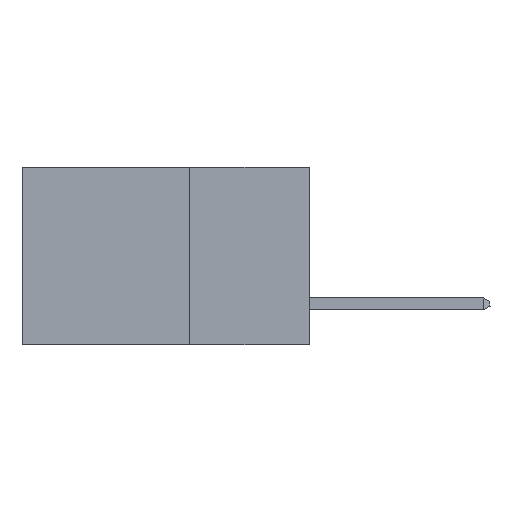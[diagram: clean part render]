
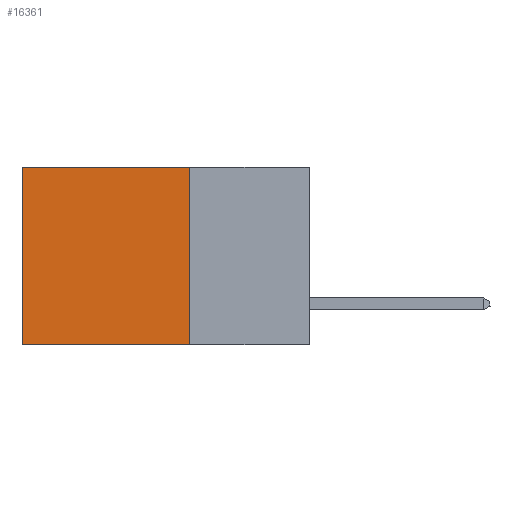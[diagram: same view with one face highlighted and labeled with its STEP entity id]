
A CAD part, left-side view. The second image highlights one B-rep face of the part: STEP entity #16361.
In plain terms, the highlighted planar face has unit normal (-1, 0, 0).
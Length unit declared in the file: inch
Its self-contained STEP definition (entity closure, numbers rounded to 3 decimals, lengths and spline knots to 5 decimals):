
#783 = VECTOR ( 'NONE', #18225, 39.37008 ) ;
#1828 = VERTEX_POINT ( 'NONE', #3755 ) ;
#2217 = EDGE_CURVE ( 'NONE', #1828, #13126, #6902, .T. ) ;
#2695 = DIRECTION ( 'NONE',  ( 0., 0., -1. ) ) ;
#3755 = CARTESIAN_POINT ( 'NONE',  ( 0.2875, 0.25, 0. ) ) ;
#3832 = ORIENTED_EDGE ( 'NONE', *, *, #2217, .F. ) ;
#5717 = EDGE_CURVE ( 'NONE', #6913, #8859, #11396, .T. ) ;
#6776 = AXIS2_PLACEMENT_3D ( 'NONE', #12167, #13519, #13450 ) ;
#6842 = DIRECTION ( 'NONE',  ( 0., 0., -1. ) ) ;
#6902 = LINE ( 'NONE', #15708, #10054 ) ;
#6913 = VERTEX_POINT ( 'NONE', #17330 ) ;
#7118 = EDGE_CURVE ( 'NONE', #1828, #6913, #10706, .T. ) ;
#8121 = CARTESIAN_POINT ( 'NONE',  ( 0.2875, 0.25, -0.37 ) ) ;
#8601 = ORIENTED_EDGE ( 'NONE', *, *, #5717, .T. ) ;
#8713 = LINE ( 'NONE', #9510, #14536 ) ;
#8859 = VERTEX_POINT ( 'NONE', #9231 ) ;
#9231 = CARTESIAN_POINT ( 'NONE',  ( 0.2875, 0.6, -0.37 ) ) ;
#9510 = CARTESIAN_POINT ( 'NONE',  ( 0.2875, 0.25, -0.37 ) ) ;
#10054 = VECTOR ( 'NONE', #2695, 39.37008 ) ;
#10706 = LINE ( 'NONE', #13238, #783 ) ;
#11093 = DIRECTION ( 'NONE',  ( 0., 1., 0. ) ) ;
#11351 = ORIENTED_EDGE ( 'NONE', *, *, #7118, .T. ) ;
#11396 = LINE ( 'NONE', #16739, #17244 ) ;
#12167 = CARTESIAN_POINT ( 'NONE',  ( 0.2875, 0.25, 0. ) ) ;
#13126 = VERTEX_POINT ( 'NONE', #8121 ) ;
#13238 = CARTESIAN_POINT ( 'NONE',  ( 0.2875, 0.25, 0. ) ) ;
#13450 = DIRECTION ( 'NONE',  ( 0., 0., -1. ) ) ;
#13519 = DIRECTION ( 'NONE',  ( 1., 0., 0. ) ) ;
#14536 = VECTOR ( 'NONE', #11093, 39.37008 ) ;
#15708 = CARTESIAN_POINT ( 'NONE',  ( 0.2875, 0.25, 0. ) ) ;
#16361 = ADVANCED_FACE ( 'NONE', ( #18614 ), #16456, .F. ) ;
#16456 = PLANE ( 'NONE',  #6776 ) ;
#16739 = CARTESIAN_POINT ( 'NONE',  ( 0.2875, 0.6, 0. ) ) ;
#17244 = VECTOR ( 'NONE', #6842, 39.37008 ) ;
#17330 = CARTESIAN_POINT ( 'NONE',  ( 0.2875, 0.6, 0. ) ) ;
#17456 = EDGE_LOOP ( 'NONE', ( #8601, #18133, #3832, #11351 ) ) ;
#17686 = EDGE_CURVE ( 'NONE', #13126, #8859, #8713, .T. ) ;
#18133 = ORIENTED_EDGE ( 'NONE', *, *, #17686, .F. ) ;
#18225 = DIRECTION ( 'NONE',  ( 0., 1., 0. ) ) ;
#18614 = FACE_OUTER_BOUND ( 'NONE', #17456, .T. ) ;
